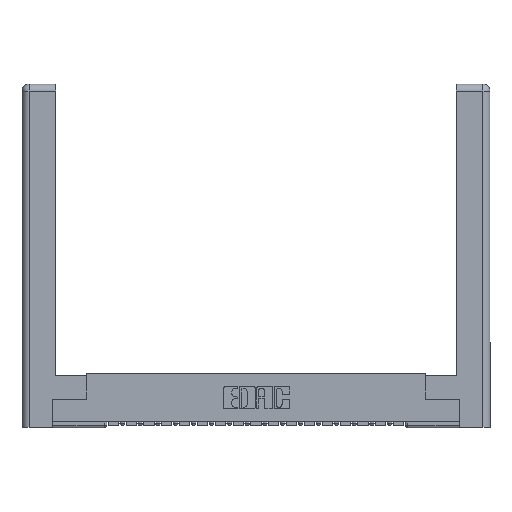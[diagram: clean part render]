
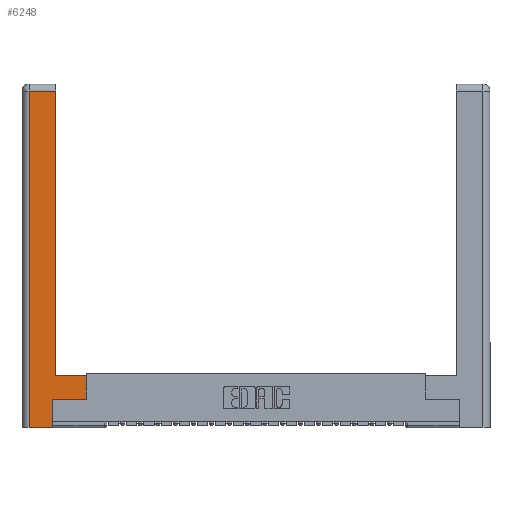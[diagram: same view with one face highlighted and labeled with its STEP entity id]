
A CAD part, top view. The second image highlights one B-rep face of the part: STEP entity #6248.
In plain terms, the highlighted planar face has unit normal (0, 0, 1).
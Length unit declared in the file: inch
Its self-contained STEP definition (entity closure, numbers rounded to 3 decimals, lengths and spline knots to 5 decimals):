
#7 = DIRECTION ( 'NONE',  ( 0., 1., 0. ) ) ;
#193 = ORIENTED_EDGE ( 'NONE', *, *, #7517, .T. ) ;
#220 = LINE ( 'NONE', #13336, #8960 ) ;
#236 = CARTESIAN_POINT ( 'NONE',  ( 0.265, 0., 0. ) ) ;
#374 = VERTEX_POINT ( 'NONE', #10954 ) ;
#1369 = LINE ( 'NONE', #14154, #4913 ) ;
#2134 = LINE ( 'NONE', #18684, #2581 ) ;
#2381 = DIRECTION ( 'NONE',  ( 0., 1., 0. ) ) ;
#2438 = VERTEX_POINT ( 'NONE', #236 ) ;
#2518 = CARTESIAN_POINT ( 'NONE',  ( 0.295, 0.45, 0. ) ) ;
#2539 = VERTEX_POINT ( 'NONE', #7533 ) ;
#2581 = VECTOR ( 'NONE', #5474, 39.37008 ) ;
#2633 = LINE ( 'NONE', #2518, #3370 ) ;
#2942 = PLANE ( 'NONE',  #18056 ) ;
#3111 = ORIENTED_EDGE ( 'NONE', *, *, #14116, .T. ) ;
#3136 = DIRECTION ( 'NONE',  ( -1., 0., 0. ) ) ;
#3156 = VERTEX_POINT ( 'NONE', #3517 ) ;
#3370 = VECTOR ( 'NONE', #15634, 39.37008 ) ;
#3517 = CARTESIAN_POINT ( 'NONE',  ( 0.295, 0.45, 0. ) ) ;
#4451 = DIRECTION ( 'NONE',  ( 0., 0., -1. ) ) ;
#4913 = VECTOR ( 'NONE', #5983, 39.37008 ) ;
#5393 = CARTESIAN_POINT ( 'NONE',  ( 0.0615, 2.94, 0. ) ) ;
#5474 = DIRECTION ( 'NONE',  ( 1., 0., 0. ) ) ;
#5983 = DIRECTION ( 'NONE',  ( 0., 1., 0. ) ) ;
#6248 = ADVANCED_FACE ( 'NONE', ( #12625 ), #2942, .F. ) ;
#7517 = EDGE_CURVE ( 'NONE', #7837, #3156, #2633, .T. ) ;
#7533 = CARTESIAN_POINT ( 'NONE',  ( 0.0615, 0., 0. ) ) ;
#7837 = VERTEX_POINT ( 'NONE', #14861 ) ;
#7977 = DIRECTION ( 'NONE',  ( -1., 0., 0. ) ) ;
#8077 = CARTESIAN_POINT ( 'NONE',  ( 0.0615, 2.94, 0. ) ) ;
#8358 = VECTOR ( 'NONE', #20897, 39.37008 ) ;
#8960 = VECTOR ( 'NONE', #7, 39.37008 ) ;
#9142 = LINE ( 'NONE', #10536, #12469 ) ;
#9593 = CARTESIAN_POINT ( 'NONE',  ( 0., 0., 0. ) ) ;
#10536 = CARTESIAN_POINT ( 'NONE',  ( 0.295, 3., 0. ) ) ;
#10628 = ORIENTED_EDGE ( 'NONE', *, *, #18794, .T. ) ;
#10748 = EDGE_LOOP ( 'NONE', ( #3111, #14669, #11298, #13634, #17502, #13584, #10628, #193 ) ) ;
#10889 = CARTESIAN_POINT ( 'NONE',  ( 0.565, 0.245, 0. ) ) ;
#10954 = CARTESIAN_POINT ( 'NONE',  ( 0.295, 2.94, 0. ) ) ;
#10976 = VERTEX_POINT ( 'NONE', #13868 ) ;
#10984 = LINE ( 'NONE', #10889, #8358 ) ;
#11298 = ORIENTED_EDGE ( 'NONE', *, *, #13369, .T. ) ;
#11457 = EDGE_CURVE ( 'NONE', #2539, #2438, #2134, .T. ) ;
#12469 = VECTOR ( 'NONE', #2381, 39.37008 ) ;
#12625 = FACE_OUTER_BOUND ( 'NONE', #10748, .T. ) ;
#12644 = LINE ( 'NONE', #19201, #14503 ) ;
#13122 = CARTESIAN_POINT ( 'NONE',  ( 0.265, 0.245, 0. ) ) ;
#13336 = CARTESIAN_POINT ( 'NONE',  ( 0.265, 0.245, 0. ) ) ;
#13369 = EDGE_CURVE ( 'NONE', #19428, #2539, #12644, .T. ) ;
#13584 = ORIENTED_EDGE ( 'NONE', *, *, #14897, .T. ) ;
#13634 = ORIENTED_EDGE ( 'NONE', *, *, #11457, .T. ) ;
#13868 = CARTESIAN_POINT ( 'NONE',  ( 0.565, 0.245, 0. ) ) ;
#14116 = EDGE_CURVE ( 'NONE', #3156, #374, #9142, .T. ) ;
#14154 = CARTESIAN_POINT ( 'NONE',  ( 0.565, 0.45, 0. ) ) ;
#14503 = VECTOR ( 'NONE', #17566, 39.37008 ) ;
#14669 = ORIENTED_EDGE ( 'NONE', *, *, #19208, .T. ) ;
#14861 = CARTESIAN_POINT ( 'NONE',  ( 0.565, 0.45, 0. ) ) ;
#14897 = EDGE_CURVE ( 'NONE', #18084, #10976, #10984, .T. ) ;
#15634 = DIRECTION ( 'NONE',  ( -1., 0., 0. ) ) ;
#17502 = ORIENTED_EDGE ( 'NONE', *, *, #18122, .T. ) ;
#17566 = DIRECTION ( 'NONE',  ( 0., -1., 0. ) ) ;
#17858 = LINE ( 'NONE', #8077, #18994 ) ;
#18056 = AXIS2_PLACEMENT_3D ( 'NONE', #9593, #4451, #7977 ) ;
#18084 = VERTEX_POINT ( 'NONE', #13122 ) ;
#18122 = EDGE_CURVE ( 'NONE', #2438, #18084, #220, .T. ) ;
#18684 = CARTESIAN_POINT ( 'NONE',  ( 0.265, 0., 0. ) ) ;
#18794 = EDGE_CURVE ( 'NONE', #10976, #7837, #1369, .T. ) ;
#18994 = VECTOR ( 'NONE', #3136, 39.37008 ) ;
#19201 = CARTESIAN_POINT ( 'NONE',  ( 0.0615, 0., 0. ) ) ;
#19208 = EDGE_CURVE ( 'NONE', #374, #19428, #17858, .T. ) ;
#19428 = VERTEX_POINT ( 'NONE', #5393 ) ;
#20897 = DIRECTION ( 'NONE',  ( 1., 0., 0. ) ) ;
